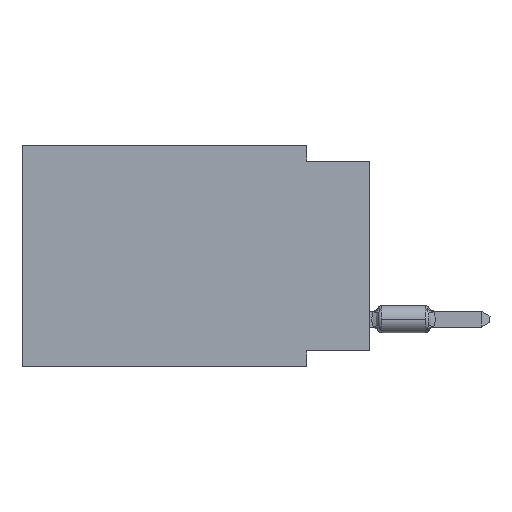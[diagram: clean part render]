
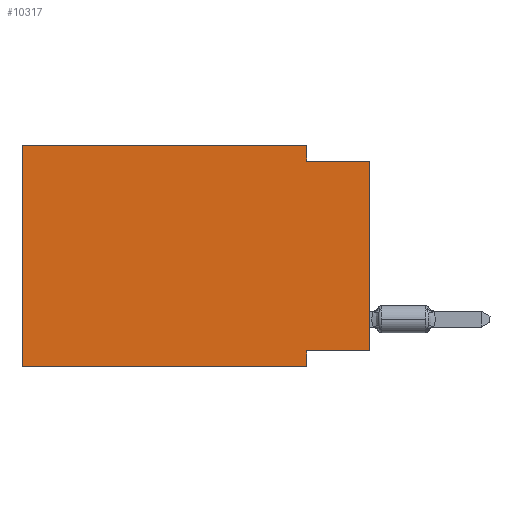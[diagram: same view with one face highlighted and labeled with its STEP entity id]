
A CAD part, left-side view. The second image highlights one B-rep face of the part: STEP entity #10317.
In plain terms, the highlighted planar face has unit normal (-1, 0, 0).
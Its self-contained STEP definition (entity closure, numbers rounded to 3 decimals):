
#22 = ORIENTED_EDGE ( 'NONE', *, *, #1510, .F. ) ;
#191 = DIRECTION ( 'NONE',  ( 0., 1., 0. ) ) ;
#260 = VERTEX_POINT ( 'NONE', #14432 ) ;
#358 = LINE ( 'NONE', #13979, #14179 ) ;
#449 = VECTOR ( 'NONE', #3733, 1000. ) ;
#600 = ORIENTED_EDGE ( 'NONE', *, *, #8680, .F. ) ;
#685 = EDGE_CURVE ( 'NONE', #260, #2782, #17820, .T. ) ;
#1002 = CARTESIAN_POINT ( 'NONE',  ( 0., 2.54, 0. ) ) ;
#1510 = EDGE_CURVE ( 'NONE', #16037, #1852, #13348, .T. ) ;
#1559 = VECTOR ( 'NONE', #6509, 1000. ) ;
#1617 = EDGE_CURVE ( 'NONE', #1852, #14431, #9902, .T. ) ;
#1786 = VECTOR ( 'NONE', #10398, 1000. ) ;
#1852 = VERTEX_POINT ( 'NONE', #9183 ) ;
#2782 = VERTEX_POINT ( 'NONE', #7213 ) ;
#3371 = FACE_OUTER_BOUND ( 'NONE', #15657, .T. ) ;
#3614 = ORIENTED_EDGE ( 'NONE', *, *, #14064, .F. ) ;
#3733 = DIRECTION ( 'NONE',  ( 0., 0., 1. ) ) ;
#4135 = CARTESIAN_POINT ( 'NONE',  ( 0., 13.97, 0. ) ) ;
#5698 = VERTEX_POINT ( 'NONE', #17655 ) ;
#6005 = CARTESIAN_POINT ( 'NONE',  ( 0., 13.97, 0. ) ) ;
#6014 = ORIENTED_EDGE ( 'NONE', *, *, #685, .F. ) ;
#6352 = CARTESIAN_POINT ( 'NONE',  ( 0., 2.54, 0. ) ) ;
#6392 = CARTESIAN_POINT ( 'NONE',  ( 0., 13.97, -8.89 ) ) ;
#6509 = DIRECTION ( 'NONE',  ( 0., 0., -1. ) ) ;
#6853 = LINE ( 'NONE', #8202, #14182 ) ;
#7213 = CARTESIAN_POINT ( 'NONE',  ( 0., 2.54, -8.89 ) ) ;
#7273 = ORIENTED_EDGE ( 'NONE', *, *, #1617, .F. ) ;
#7437 = PLANE ( 'NONE',  #10265 ) ;
#7609 = VECTOR ( 'NONE', #7904, 1000. ) ;
#7759 = EDGE_CURVE ( 'NONE', #5698, #260, #358, .T. ) ;
#7904 = DIRECTION ( 'NONE',  ( 0., 0., -1. ) ) ;
#7993 = CARTESIAN_POINT ( 'NONE',  ( 0., 2.54, -8.89 ) ) ;
#8202 = CARTESIAN_POINT ( 'NONE',  ( 0., 13.97, -8.89 ) ) ;
#8680 = EDGE_CURVE ( 'NONE', #11976, #16037, #15648, .T. ) ;
#9147 = CARTESIAN_POINT ( 'NONE',  ( 0., 0., 0. ) ) ;
#9183 = CARTESIAN_POINT ( 'NONE',  ( 0., 2.54, -0.635 ) ) ;
#9243 = EDGE_CURVE ( 'NONE', #12684, #2782, #6853, .T. ) ;
#9902 = LINE ( 'NONE', #15054, #15968 ) ;
#10265 = AXIS2_PLACEMENT_3D ( 'NONE', #14277, #10382, #15892 ) ;
#10317 = ADVANCED_FACE ( 'NONE', ( #3371 ), #7437, .F. ) ;
#10382 = DIRECTION ( 'NONE',  ( 1., 0., 0. ) ) ;
#10398 = DIRECTION ( 'NONE',  ( 0., -1., 0. ) ) ;
#10584 = LINE ( 'NONE', #9147, #449 ) ;
#10804 = DIRECTION ( 'NONE',  ( 0., 0., 1. ) ) ;
#11163 = LINE ( 'NONE', #4135, #15716 ) ;
#11938 = CARTESIAN_POINT ( 'NONE',  ( 0., 13.97, 0. ) ) ;
#11976 = VERTEX_POINT ( 'NONE', #11938 ) ;
#12684 = VERTEX_POINT ( 'NONE', #6392 ) ;
#12884 = ORIENTED_EDGE ( 'NONE', *, *, #9243, .T. ) ;
#13348 = LINE ( 'NONE', #1002, #1559 ) ;
#13486 = CARTESIAN_POINT ( 'NONE',  ( 0., 0., -0.635 ) ) ;
#13527 = EDGE_CURVE ( 'NONE', #5698, #14431, #10584, .T. ) ;
#13979 = CARTESIAN_POINT ( 'NONE',  ( 0., 0., -8.255 ) ) ;
#14064 = EDGE_CURVE ( 'NONE', #12684, #11976, #11163, .T. ) ;
#14179 = VECTOR ( 'NONE', #191, 1000. ) ;
#14182 = VECTOR ( 'NONE', #17584, 1000. ) ;
#14277 = CARTESIAN_POINT ( 'NONE',  ( 0., 13.97, 0. ) ) ;
#14431 = VERTEX_POINT ( 'NONE', #13486 ) ;
#14432 = CARTESIAN_POINT ( 'NONE',  ( 0., 2.54, -8.255 ) ) ;
#15054 = CARTESIAN_POINT ( 'NONE',  ( 0., 0., -0.635 ) ) ;
#15318 = DIRECTION ( 'NONE',  ( 0., -1., 0. ) ) ;
#15648 = LINE ( 'NONE', #6005, #1786 ) ;
#15657 = EDGE_LOOP ( 'NONE', ( #17609, #7273, #22, #600, #3614, #12884, #6014, #16082 ) ) ;
#15716 = VECTOR ( 'NONE', #10804, 1000. ) ;
#15892 = DIRECTION ( 'NONE',  ( 0., 0., -1. ) ) ;
#15968 = VECTOR ( 'NONE', #15318, 1000. ) ;
#16037 = VERTEX_POINT ( 'NONE', #6352 ) ;
#16082 = ORIENTED_EDGE ( 'NONE', *, *, #7759, .F. ) ;
#17584 = DIRECTION ( 'NONE',  ( 0., -1., 0. ) ) ;
#17609 = ORIENTED_EDGE ( 'NONE', *, *, #13527, .T. ) ;
#17655 = CARTESIAN_POINT ( 'NONE',  ( 0., 0., -8.255 ) ) ;
#17820 = LINE ( 'NONE', #7993, #7609 ) ;
